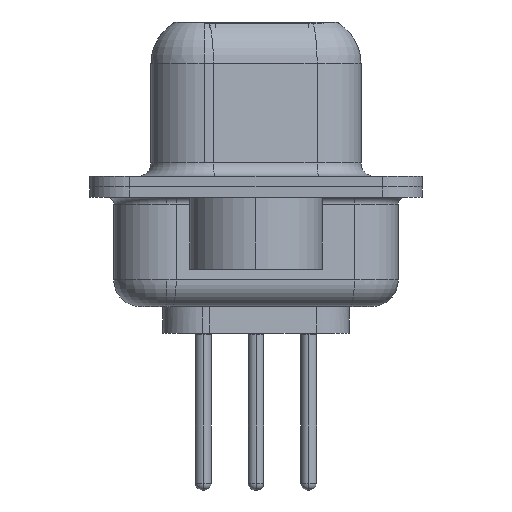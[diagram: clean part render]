
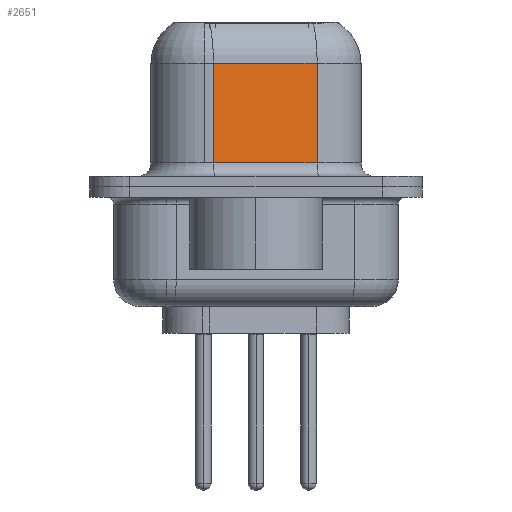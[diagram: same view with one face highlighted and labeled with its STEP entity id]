
A CAD part, left-side view. The second image highlights one B-rep face of the part: STEP entity #2651.
In plain terms, the highlighted planar face has unit normal (-0.985, -0.174, 0).
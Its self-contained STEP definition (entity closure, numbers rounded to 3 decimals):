
#919 = EDGE_LOOP ( 'NONE', ( #22863, #6936, #13150, #8524 ) ) ;
#1711 = CARTESIAN_POINT ( 'NONE',  ( 5.043, -2.297, 0.9 ) ) ;
#1805 = EDGE_CURVE ( 'NONE', #27937, #12057, #28106, .T. ) ;
#2027 = AXIS2_PLACEMENT_3D ( 'NONE', #11829, #4989, #5154 ) ;
#2163 = VECTOR ( 'NONE', #19402, 1000. ) ;
#2651 = ADVANCED_FACE ( 'NONE', ( #2843 ), #26235, .F. ) ;
#2694 = VERTEX_POINT ( 'NONE', #7468 ) ;
#2843 = FACE_OUTER_BOUND ( 'NONE', #919, .T. ) ;
#3895 = VECTOR ( 'NONE', #17160, 1000. ) ;
#4989 = DIRECTION ( 'NONE',  ( 0.985, 0.174, 0. ) ) ;
#5154 = DIRECTION ( 'NONE',  ( -0.174, 0.985, 0. ) ) ;
#6936 = ORIENTED_EDGE ( 'NONE', *, *, #1805, .T. ) ;
#7468 = CARTESIAN_POINT ( 'NONE',  ( 4.355, 1.603, 0.9 ) ) ;
#7707 = CARTESIAN_POINT ( 'NONE',  ( 5.043, -2.297, 6.4 ) ) ;
#8524 = ORIENTED_EDGE ( 'NONE', *, *, #21683, .T. ) ;
#9736 = DIRECTION ( 'NONE',  ( 0.174, -0.985, 0. ) ) ;
#11829 = CARTESIAN_POINT ( 'NONE',  ( 5.043, -2.297, 6.4 ) ) ;
#12057 = VERTEX_POINT ( 'NONE', #24353 ) ;
#12795 = CARTESIAN_POINT ( 'NONE',  ( 4.355, 1.603, 6.4 ) ) ;
#13150 = ORIENTED_EDGE ( 'NONE', *, *, #23407, .T. ) ;
#14616 = CARTESIAN_POINT ( 'NONE',  ( 5.043, -2.297, 4.65 ) ) ;
#16390 = LINE ( 'NONE', #25855, #26877 ) ;
#17160 = DIRECTION ( 'NONE',  ( 0., 0., -1. ) ) ;
#17653 = CARTESIAN_POINT ( 'NONE',  ( 5.043, -2.297, 4.65 ) ) ;
#17749 = DIRECTION ( 'NONE',  ( 0., 0., -1. ) ) ;
#18232 = VERTEX_POINT ( 'NONE', #1711 ) ;
#19402 = DIRECTION ( 'NONE',  ( -0.174, 0.985, 0. ) ) ;
#21683 = EDGE_CURVE ( 'NONE', #2694, #18232, #16390, .T. ) ;
#22863 = ORIENTED_EDGE ( 'NONE', *, *, #28254, .F. ) ;
#23407 = EDGE_CURVE ( 'NONE', #12057, #2694, #25190, .T. ) ;
#24353 = CARTESIAN_POINT ( 'NONE',  ( 4.355, 1.603, 4.65 ) ) ;
#25190 = LINE ( 'NONE', #12795, #27343 ) ;
#25855 = CARTESIAN_POINT ( 'NONE',  ( 5.043, -2.297, 0.9 ) ) ;
#26235 = PLANE ( 'NONE',  #2027 ) ;
#26877 = VECTOR ( 'NONE', #9736, 1000. ) ;
#27343 = VECTOR ( 'NONE', #17749, 1000. ) ;
#27937 = VERTEX_POINT ( 'NONE', #17653 ) ;
#28106 = LINE ( 'NONE', #14616, #2163 ) ;
#28254 = EDGE_CURVE ( 'NONE', #27937, #18232, #28924, .T. ) ;
#28924 = LINE ( 'NONE', #7707, #3895 ) ;
